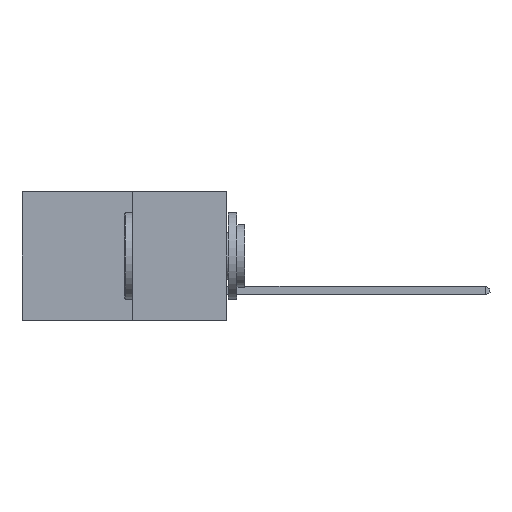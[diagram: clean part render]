
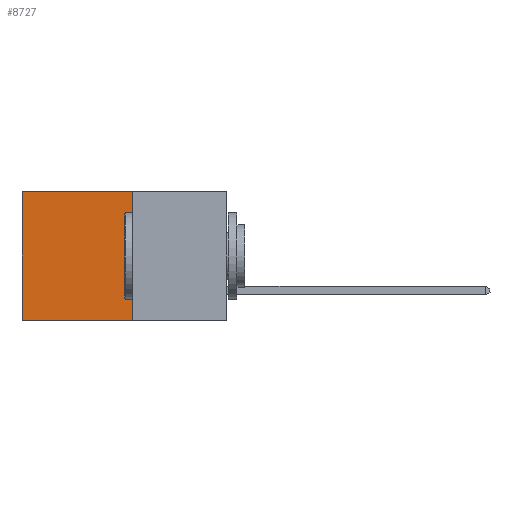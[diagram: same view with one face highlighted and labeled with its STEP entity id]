
A CAD part, left-side view. The second image highlights one B-rep face of the part: STEP entity #8727.
In plain terms, the highlighted planar face has unit normal (-1, 0, 0).
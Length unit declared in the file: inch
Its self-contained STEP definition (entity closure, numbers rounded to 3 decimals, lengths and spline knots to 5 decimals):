
#218 = EDGE_CURVE ( 'NONE', #7963, #9277, #4226, .T. ) ;
#409 = DIRECTION ( 'NONE',  ( 0., 0., -1. ) ) ;
#424 = CARTESIAN_POINT ( 'NONE',  ( 0.277, 0.59, -0.37 ) ) ;
#621 = LINE ( 'NONE', #424, #6580 ) ;
#1027 = CARTESIAN_POINT ( 'NONE',  ( 0.277, 0.27, -0.37 ) ) ;
#1048 = CARTESIAN_POINT ( 'NONE',  ( 0.277, 0.59, 0. ) ) ;
#1090 = CARTESIAN_POINT ( 'NONE',  ( 0.277, 0.27, -0.37 ) ) ;
#1743 = EDGE_CURVE ( 'NONE', #9277, #5391, #621, .T. ) ;
#1915 = DIRECTION ( 'NONE',  ( 0., 0., -1. ) ) ;
#2117 = ORIENTED_EDGE ( 'NONE', *, *, #1743, .T. ) ;
#2266 = CARTESIAN_POINT ( 'NONE',  ( 0.277, 0.27, 0. ) ) ;
#3399 = CARTESIAN_POINT ( 'NONE',  ( 0.277, 0.27, 0. ) ) ;
#3504 = VERTEX_POINT ( 'NONE', #3660 ) ;
#3660 = CARTESIAN_POINT ( 'NONE',  ( 0.277, 0.27, -0.37 ) ) ;
#4123 = DIRECTION ( 'NONE',  ( 0., 1., 0. ) ) ;
#4226 = LINE ( 'NONE', #2266, #9475 ) ;
#4410 = ORIENTED_EDGE ( 'NONE', *, *, #6055, .F. ) ;
#4583 = FACE_OUTER_BOUND ( 'NONE', #5192, .T. ) ;
#5192 = EDGE_LOOP ( 'NONE', ( #2117, #4410, #6906, #7352 ) ) ;
#5391 = VERTEX_POINT ( 'NONE', #8846 ) ;
#5696 = DIRECTION ( 'NONE',  ( 0., 0., -1. ) ) ;
#5765 = PLANE ( 'NONE',  #8947 ) ;
#5950 = DIRECTION ( 'NONE',  ( 0., 1., 0. ) ) ;
#6055 = EDGE_CURVE ( 'NONE', #3504, #5391, #9010, .T. ) ;
#6512 = DIRECTION ( 'NONE',  ( 1., 0., 0. ) ) ;
#6580 = VECTOR ( 'NONE', #409, 39.37008 ) ;
#6906 = ORIENTED_EDGE ( 'NONE', *, *, #7980, .F. ) ;
#7017 = LINE ( 'NONE', #1027, #8511 ) ;
#7352 = ORIENTED_EDGE ( 'NONE', *, *, #218, .T. ) ;
#7963 = VERTEX_POINT ( 'NONE', #3399 ) ;
#7980 = EDGE_CURVE ( 'NONE', #7963, #3504, #7017, .T. ) ;
#8511 = VECTOR ( 'NONE', #5696, 39.37008 ) ;
#8597 = CARTESIAN_POINT ( 'NONE',  ( 0.277, 0.27, -0.37 ) ) ;
#8727 = ADVANCED_FACE ( 'NONE', ( #4583 ), #5765, .F. ) ;
#8846 = CARTESIAN_POINT ( 'NONE',  ( 0.277, 0.59, -0.37 ) ) ;
#8947 = AXIS2_PLACEMENT_3D ( 'NONE', #1090, #6512, #1915 ) ;
#9010 = LINE ( 'NONE', #8597, #9231 ) ;
#9231 = VECTOR ( 'NONE', #4123, 39.37008 ) ;
#9277 = VERTEX_POINT ( 'NONE', #1048 ) ;
#9475 = VECTOR ( 'NONE', #5950, 39.37008 ) ;
